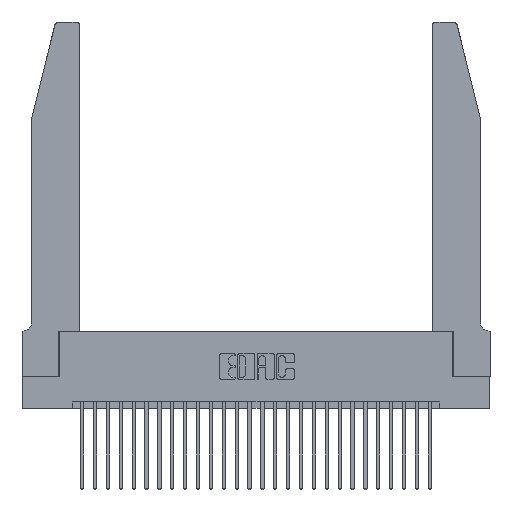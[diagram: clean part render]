
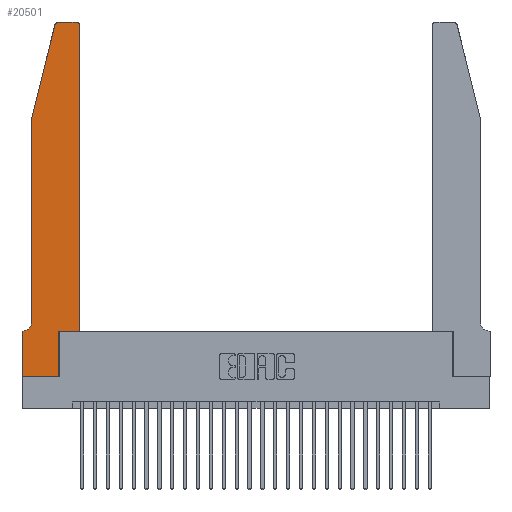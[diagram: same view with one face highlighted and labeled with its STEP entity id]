
A CAD part, top view. The second image highlights one B-rep face of the part: STEP entity #20501.
In plain terms, the highlighted planar face has unit normal (0, 0, 1).
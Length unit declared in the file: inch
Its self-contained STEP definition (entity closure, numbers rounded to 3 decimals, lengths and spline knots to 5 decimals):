
#497 = VERTEX_POINT ( 'NONE', #1586 ) ;
#688 = LINE ( 'NONE', #23527, #10369 ) ;
#794 = CARTESIAN_POINT ( 'NONE',  ( 0.0055, 0.35, 0.37 ) ) ;
#853 = EDGE_CURVE ( 'NONE', #23830, #20225, #25612, .T. ) ;
#975 = CIRCLE ( 'NONE', #28389, 0.03 ) ;
#1193 = CARTESIAN_POINT ( 'NONE',  ( 0.4505, 2.72, 0.37 ) ) ;
#1287 = EDGE_CURVE ( 'NONE', #6401, #23830, #23193, .T. ) ;
#1586 = CARTESIAN_POINT ( 'NONE',  ( 0.0755, 2., 0.37 ) ) ;
#2125 = DIRECTION ( 'NONE',  ( 0., 0., -1. ) ) ;
#2586 = LINE ( 'NONE', #19943, #13636 ) ;
#2699 = ORIENTED_EDGE ( 'NONE', *, *, #12047, .T. ) ;
#2931 = VERTEX_POINT ( 'NONE', #11650 ) ;
#3807 = CARTESIAN_POINT ( 'NONE',  ( 0., 0., 0.37 ) ) ;
#3894 = CARTESIAN_POINT ( 'NONE',  ( 0.2605, 2.75, 0.37 ) ) ;
#4489 = VECTOR ( 'NONE', #26422, 39.37008 ) ;
#4545 = DIRECTION ( 'NONE',  ( 0., 0., 1. ) ) ;
#4734 = AXIS2_PLACEMENT_3D ( 'NONE', #21885, #2125, #26510 ) ;
#4755 = EDGE_CURVE ( 'NONE', #25459, #9425, #14639, .T. ) ;
#5166 = AXIS2_PLACEMENT_3D ( 'NONE', #19218, #14767, #6073 ) ;
#5904 = ORIENTED_EDGE ( 'NONE', *, *, #4755, .T. ) ;
#6069 = EDGE_CURVE ( 'NONE', #19874, #25459, #25642, .T. ) ;
#6073 = DIRECTION ( 'NONE',  ( 1., 0., 0. ) ) ;
#6401 = VERTEX_POINT ( 'NONE', #20560 ) ;
#6421 = DIRECTION ( 'NONE',  ( 1., 0., 0. ) ) ;
#6563 = ORIENTED_EDGE ( 'NONE', *, *, #17366, .T. ) ;
#6991 = DIRECTION ( 'NONE',  ( 0., -1., 0. ) ) ;
#7289 = VERTEX_POINT ( 'NONE', #794 ) ;
#7885 = EDGE_CURVE ( 'NONE', #9425, #24715, #26291, .T. ) ;
#8216 = DIRECTION ( 'NONE',  ( -0.239, -0.971, 0. ) ) ;
#8268 = ORIENTED_EDGE ( 'NONE', *, *, #6069, .T. ) ;
#9038 = DIRECTION ( 'NONE',  ( -1., 0., 0. ) ) ;
#9261 = VECTOR ( 'NONE', #11218, 39.37008 ) ;
#9425 = VERTEX_POINT ( 'NONE', #17658 ) ;
#9814 = ORIENTED_EDGE ( 'NONE', *, *, #26728, .T. ) ;
#10369 = VECTOR ( 'NONE', #8216, 39.37008 ) ;
#10849 = ORIENTED_EDGE ( 'NONE', *, *, #14503, .T. ) ;
#11025 = FACE_OUTER_BOUND ( 'NONE', #11172, .T. ) ;
#11089 = ORIENTED_EDGE ( 'NONE', *, *, #13190, .T. ) ;
#11099 = VERTEX_POINT ( 'NONE', #12549 ) ;
#11172 = EDGE_LOOP ( 'NONE', ( #23124, #14089, #17314, #10849, #6563, #11089, #9814, #24303, #8268, #5904, #22522, #2699 ) ) ;
#11218 = DIRECTION ( 'NONE',  ( 1., 0., 0. ) ) ;
#11451 = CARTESIAN_POINT ( 'NONE',  ( 0.0755, 0.35, 0.37 ) ) ;
#11616 = CARTESIAN_POINT ( 'NONE',  ( 0.4505, 0.35, 0.37 ) ) ;
#11650 = CARTESIAN_POINT ( 'NONE',  ( 0.0755, 0.42, 0.37 ) ) ;
#12047 = EDGE_CURVE ( 'NONE', #24715, #6401, #975, .T. ) ;
#12105 = EDGE_CURVE ( 'NONE', #18711, #19874, #15837, .T. ) ;
#12539 = CARTESIAN_POINT ( 'NONE',  ( 0.2865, 0.35, 0.37 ) ) ;
#12549 = CARTESIAN_POINT ( 'NONE',  ( 0., 0.35, 0.37 ) ) ;
#13153 = CARTESIAN_POINT ( 'NONE',  ( 0., 0., 0.37 ) ) ;
#13190 = EDGE_CURVE ( 'NONE', #7289, #11099, #18536, .T. ) ;
#13245 = DIRECTION ( 'NONE',  ( 1., 0., 0. ) ) ;
#13636 = VECTOR ( 'NONE', #6991, 39.37008 ) ;
#13679 = CARTESIAN_POINT ( 'NONE',  ( 0.2865, 0., 0.37 ) ) ;
#14089 = ORIENTED_EDGE ( 'NONE', *, *, #853, .T. ) ;
#14503 = EDGE_CURVE ( 'NONE', #497, #2931, #2586, .T. ) ;
#14639 = LINE ( 'NONE', #11616, #22994 ) ;
#14767 = DIRECTION ( 'NONE',  ( 0., 0., 1. ) ) ;
#15538 = VECTOR ( 'NONE', #22734, 39.37008 ) ;
#15837 = LINE ( 'NONE', #13153, #9261 ) ;
#15958 = VECTOR ( 'NONE', #21070, 39.37008 ) ;
#17004 = PLANE ( 'NONE',  #5166 ) ;
#17314 = ORIENTED_EDGE ( 'NONE', *, *, #27500, .T. ) ;
#17366 = EDGE_CURVE ( 'NONE', #2931, #7289, #18277, .T. ) ;
#17658 = CARTESIAN_POINT ( 'NONE',  ( 0.4505, 0.35, 0.37 ) ) ;
#18277 = CIRCLE ( 'NONE', #4734, 0.07 ) ;
#18536 = LINE ( 'NONE', #11451, #19258 ) ;
#18711 = VERTEX_POINT ( 'NONE', #24495 ) ;
#19182 = DIRECTION ( 'NONE',  ( 0., -1., 0. ) ) ;
#19218 = CARTESIAN_POINT ( 'NONE',  ( 0., 0.35, 0.37 ) ) ;
#19258 = VECTOR ( 'NONE', #9038, 39.37008 ) ;
#19874 = VERTEX_POINT ( 'NONE', #13679 ) ;
#19943 = CARTESIAN_POINT ( 'NONE',  ( 0.0755, 2., 0.37 ) ) ;
#20113 = LINE ( 'NONE', #3807, #25302 ) ;
#20225 = VERTEX_POINT ( 'NONE', #22177 ) ;
#20501 = ADVANCED_FACE ( 'NONE', ( #11025 ), #17004, .T. ) ;
#20560 = CARTESIAN_POINT ( 'NONE',  ( 0.4205, 2.75, 0.37 ) ) ;
#21070 = DIRECTION ( 'NONE',  ( 0., 1., 0. ) ) ;
#21571 = CARTESIAN_POINT ( 'NONE',  ( 0.284, 2.75, 0.37 ) ) ;
#21885 = CARTESIAN_POINT ( 'NONE',  ( 0.0055, 0.42, 0.37 ) ) ;
#22177 = CARTESIAN_POINT ( 'NONE',  ( 0.25487, 2.72718, 0.37 ) ) ;
#22522 = ORIENTED_EDGE ( 'NONE', *, *, #7885, .T. ) ;
#22734 = DIRECTION ( 'NONE',  ( 0., 1., 0. ) ) ;
#22994 = VECTOR ( 'NONE', #27195, 39.37008 ) ;
#23124 = ORIENTED_EDGE ( 'NONE', *, *, #1287, .T. ) ;
#23193 = LINE ( 'NONE', #3894, #4489 ) ;
#23266 = AXIS2_PLACEMENT_3D ( 'NONE', #23280, #23371, #6421 ) ;
#23280 = CARTESIAN_POINT ( 'NONE',  ( 0.284, 2.72, 0.37 ) ) ;
#23371 = DIRECTION ( 'NONE',  ( 0., 0., 1. ) ) ;
#23527 = CARTESIAN_POINT ( 'NONE',  ( 0.0755, 2., 0.37 ) ) ;
#23830 = VERTEX_POINT ( 'NONE', #21571 ) ;
#24303 = ORIENTED_EDGE ( 'NONE', *, *, #12105, .T. ) ;
#24495 = CARTESIAN_POINT ( 'NONE',  ( 0., 0., 0.37 ) ) ;
#24715 = VERTEX_POINT ( 'NONE', #1193 ) ;
#25302 = VECTOR ( 'NONE', #19182, 39.37008 ) ;
#25341 = CARTESIAN_POINT ( 'NONE',  ( 0.2865, 0.35, 0.37 ) ) ;
#25459 = VERTEX_POINT ( 'NONE', #25341 ) ;
#25612 = CIRCLE ( 'NONE', #23266, 0.03 ) ;
#25642 = LINE ( 'NONE', #12539, #15958 ) ;
#26291 = LINE ( 'NONE', #27244, #15538 ) ;
#26422 = DIRECTION ( 'NONE',  ( -1., 0., 0. ) ) ;
#26510 = DIRECTION ( 'NONE',  ( -1., 0., 0. ) ) ;
#26710 = CARTESIAN_POINT ( 'NONE',  ( 0.4205, 2.72, 0.37 ) ) ;
#26728 = EDGE_CURVE ( 'NONE', #11099, #18711, #20113, .T. ) ;
#27195 = DIRECTION ( 'NONE',  ( 1., 0., 0. ) ) ;
#27244 = CARTESIAN_POINT ( 'NONE',  ( 0.4505, 0.35, 0.37 ) ) ;
#27500 = EDGE_CURVE ( 'NONE', #20225, #497, #688, .T. ) ;
#28389 = AXIS2_PLACEMENT_3D ( 'NONE', #26710, #4545, #13245 ) ;
